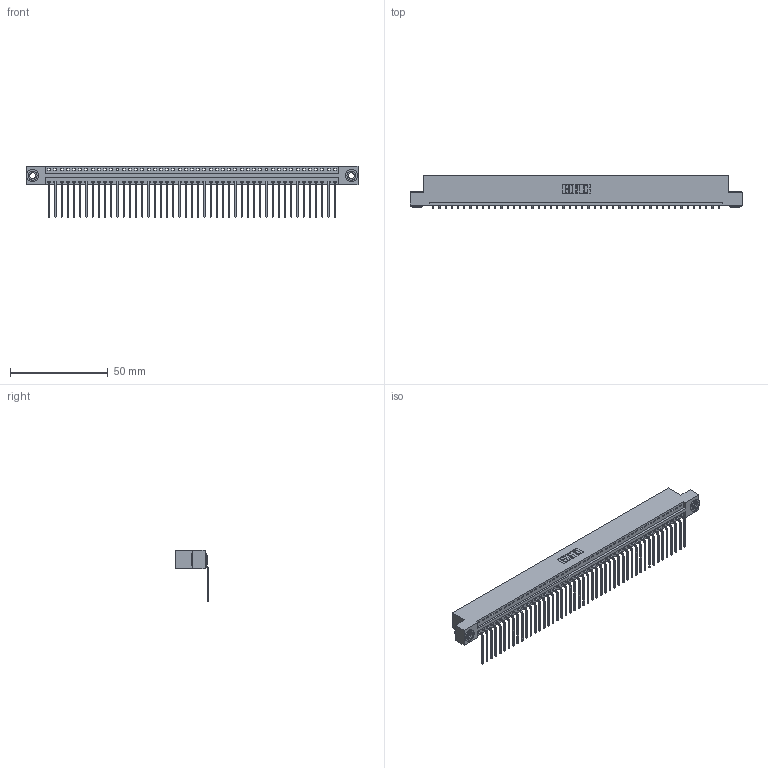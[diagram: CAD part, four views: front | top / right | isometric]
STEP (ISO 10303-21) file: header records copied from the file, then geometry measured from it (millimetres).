
FILE_DESCRIPTION (( 'STEP AP203' ), '1' );
FILE_NAME ('346-047-559-103.STEP', '2022-05-09T22:30:02', ( '' ), ( '' ), 'SwSTEP 2.0', 'SolidWorks 2020', '' );
FILE_SCHEMA (( 'CONFIG_CONTROL_DESIGN' ));
Length unit declared in the file: inch
Products named in the file (4): 345-292-001_558 559 Tail - 1; 346 Part_Flush Mounting Lugs - 0.156 Dia-TH; 345-250-002_345-250-002-102; 346-047-559-103
Assembly tree (50 placements, depth 2):
  346-047-559-103
    346 Part_Flush Mounting Lugs - 0.156 Dia-TH
    345-292-001_558 559 Tail - 1  x47
    345-250-002_345-250-002-102  x2
Bounding box: 169.8 x 17.08 x 26.16 mm (x, y, z)
Volume: 16445.9 mm3; surface area: 21794.8 mm2
Topology: 50 solids, 50 shells, 2994 faces, 8995 edges, 5930 vertices
Faces by surface type: plane 2074, cylinder 912, cone 8
Entity records: 29646 total; most frequent: CARTESIAN_POINT 5062, ORIENTED_EDGE 5034, DIRECTION 4489, EDGE_CURVE 2517, VECTOR 2173, LINE 2173, VERTEX_POINT 1674, AXIS2_PLACEMENT_3D 1158
